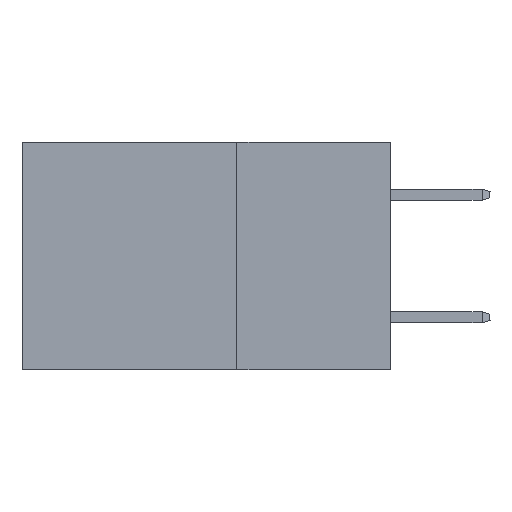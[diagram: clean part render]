
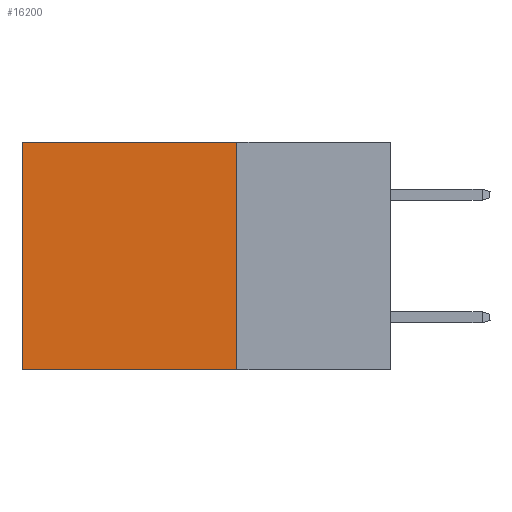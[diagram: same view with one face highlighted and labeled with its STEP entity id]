
A CAD part, left-side view. The second image highlights one B-rep face of the part: STEP entity #16200.
In plain terms, the highlighted planar face has unit normal (-1, 0, 0).
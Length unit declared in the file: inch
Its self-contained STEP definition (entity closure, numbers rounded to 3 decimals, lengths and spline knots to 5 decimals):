
#156 = CARTESIAN_POINT ( 'NONE',  ( 0.2875, 0.6, -0.37 ) ) ;
#735 = ORIENTED_EDGE ( 'NONE', *, *, #31162, .T. ) ;
#891 = ORIENTED_EDGE ( 'NONE', *, *, #2170, .F. ) ;
#1175 = CARTESIAN_POINT ( 'NONE',  ( 0.2875, 0.25, 0. ) ) ;
#1856 = LINE ( 'NONE', #3557, #10923 ) ;
#2170 = EDGE_CURVE ( 'NONE', #35563, #11371, #15343, .T. ) ;
#3557 = CARTESIAN_POINT ( 'NONE',  ( 0.2875, 0.25, 0. ) ) ;
#4537 = ORIENTED_EDGE ( 'NONE', *, *, #13859, .F. ) ;
#5095 = EDGE_LOOP ( 'NONE', ( #735, #891, #4537, #7801 ) ) ;
#6424 = DIRECTION ( 'NONE',  ( 0., 0., -1. ) ) ;
#7801 = ORIENTED_EDGE ( 'NONE', *, *, #10866, .T. ) ;
#8854 = CARTESIAN_POINT ( 'NONE',  ( 0.2875, 0.25, 0. ) ) ;
#10476 = LINE ( 'NONE', #25958, #28579 ) ;
#10866 = EDGE_CURVE ( 'NONE', #26958, #17426, #1856, .T. ) ;
#10923 = VECTOR ( 'NONE', #14166, 39.37008 ) ;
#11371 = VERTEX_POINT ( 'NONE', #156 ) ;
#13859 = EDGE_CURVE ( 'NONE', #26958, #35563, #15897, .T. ) ;
#14166 = DIRECTION ( 'NONE',  ( 0., 1., 0. ) ) ;
#15343 = LINE ( 'NONE', #21045, #25691 ) ;
#15897 = LINE ( 'NONE', #1175, #35273 ) ;
#16200 = ADVANCED_FACE ( 'NONE', ( #24250 ), #19332, .F. ) ;
#17426 = VERTEX_POINT ( 'NONE', #22470 ) ;
#19332 = PLANE ( 'NONE',  #33115 ) ;
#19699 = DIRECTION ( 'NONE',  ( 1., 0., 0. ) ) ;
#21045 = CARTESIAN_POINT ( 'NONE',  ( 0.2875, 0.25, -0.37 ) ) ;
#22470 = CARTESIAN_POINT ( 'NONE',  ( 0.2875, 0.6, 0. ) ) ;
#24250 = FACE_OUTER_BOUND ( 'NONE', #5095, .T. ) ;
#25691 = VECTOR ( 'NONE', #29311, 39.37008 ) ;
#25958 = CARTESIAN_POINT ( 'NONE',  ( 0.2875, 0.6, 0. ) ) ;
#26958 = VERTEX_POINT ( 'NONE', #8854 ) ;
#28400 = DIRECTION ( 'NONE',  ( 0., 0., -1. ) ) ;
#28579 = VECTOR ( 'NONE', #33918, 39.37008 ) ;
#29311 = DIRECTION ( 'NONE',  ( 0., 1., 0. ) ) ;
#30646 = CARTESIAN_POINT ( 'NONE',  ( 0.2875, 0.25, -0.37 ) ) ;
#31162 = EDGE_CURVE ( 'NONE', #17426, #11371, #10476, .T. ) ;
#33115 = AXIS2_PLACEMENT_3D ( 'NONE', #33164, #19699, #6424 ) ;
#33164 = CARTESIAN_POINT ( 'NONE',  ( 0.2875, 0.25, 0. ) ) ;
#33918 = DIRECTION ( 'NONE',  ( 0., 0., -1. ) ) ;
#35273 = VECTOR ( 'NONE', #28400, 39.37008 ) ;
#35563 = VERTEX_POINT ( 'NONE', #30646 ) ;
